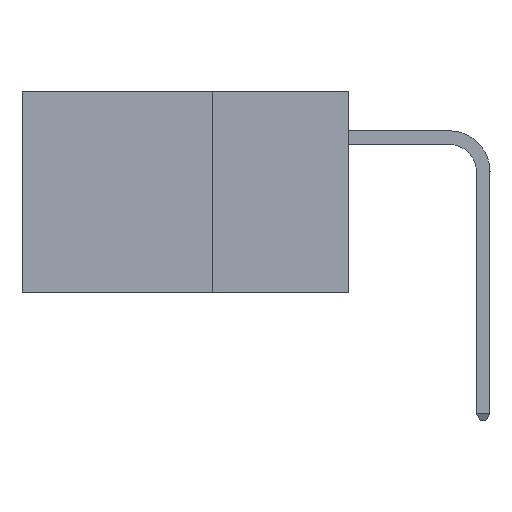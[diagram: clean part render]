
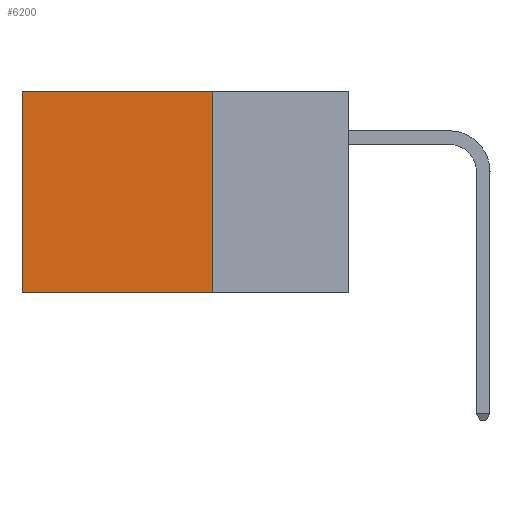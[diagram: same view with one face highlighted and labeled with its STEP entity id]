
A CAD part, left-side view. The second image highlights one B-rep face of the part: STEP entity #6200.
In plain terms, the highlighted planar face has unit normal (-1, 0, 0).
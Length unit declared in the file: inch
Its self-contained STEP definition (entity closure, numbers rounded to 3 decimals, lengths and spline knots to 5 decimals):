
#117 = VECTOR ( 'NONE', #3952, 39.37008 ) ;
#334 = PLANE ( 'NONE',  #3367 ) ;
#477 = FACE_OUTER_BOUND ( 'NONE', #5718, .T. ) ;
#944 = CARTESIAN_POINT ( 'NONE',  ( 0.2875, 0.25, 0. ) ) ;
#2582 = LINE ( 'NONE', #9122, #117 ) ;
#2603 = LINE ( 'NONE', #2713, #8702 ) ;
#2713 = CARTESIAN_POINT ( 'NONE',  ( 0.2875, 0.25, 0. ) ) ;
#2733 = CARTESIAN_POINT ( 'NONE',  ( 0.2875, 0.6, 0. ) ) ;
#2866 = LINE ( 'NONE', #10944, #5875 ) ;
#2928 = ORIENTED_EDGE ( 'NONE', *, *, #10273, .F. ) ;
#2999 = DIRECTION ( 'NONE',  ( 0., 0., -1. ) ) ;
#3357 = EDGE_CURVE ( 'NONE', #4830, #9668, #2582, .T. ) ;
#3367 = AXIS2_PLACEMENT_3D ( 'NONE', #944, #7029, #9924 ) ;
#3760 = ORIENTED_EDGE ( 'NONE', *, *, #9177, .T. ) ;
#3815 = CARTESIAN_POINT ( 'NONE',  ( 0.2875, 0.25, -0.37 ) ) ;
#3893 = ORIENTED_EDGE ( 'NONE', *, *, #7838, .F. ) ;
#3900 = DIRECTION ( 'NONE',  ( 0., 1., 0. ) ) ;
#3952 = DIRECTION ( 'NONE',  ( 0., 0., -1. ) ) ;
#4043 = ORIENTED_EDGE ( 'NONE', *, *, #3357, .T. ) ;
#4568 = DIRECTION ( 'NONE',  ( 0., 1., 0. ) ) ;
#4830 = VERTEX_POINT ( 'NONE', #2733 ) ;
#5718 = EDGE_LOOP ( 'NONE', ( #4043, #2928, #3893, #3760 ) ) ;
#5875 = VECTOR ( 'NONE', #3900, 39.37008 ) ;
#5929 = VECTOR ( 'NONE', #2999, 39.37008 ) ;
#6200 = ADVANCED_FACE ( 'NONE', ( #477 ), #334, .F. ) ;
#7029 = DIRECTION ( 'NONE',  ( 1., 0., 0. ) ) ;
#7339 = VERTEX_POINT ( 'NONE', #7905 ) ;
#7521 = VERTEX_POINT ( 'NONE', #3815 ) ;
#7642 = CARTESIAN_POINT ( 'NONE',  ( 0.2875, 0.6, -0.37 ) ) ;
#7838 = EDGE_CURVE ( 'NONE', #7339, #7521, #9569, .T. ) ;
#7905 = CARTESIAN_POINT ( 'NONE',  ( 0.2875, 0.25, 0. ) ) ;
#8702 = VECTOR ( 'NONE', #4568, 39.37008 ) ;
#9122 = CARTESIAN_POINT ( 'NONE',  ( 0.2875, 0.6, 0. ) ) ;
#9177 = EDGE_CURVE ( 'NONE', #7339, #4830, #2603, .T. ) ;
#9569 = LINE ( 'NONE', #10785, #5929 ) ;
#9668 = VERTEX_POINT ( 'NONE', #7642 ) ;
#9924 = DIRECTION ( 'NONE',  ( 0., 0., -1. ) ) ;
#10273 = EDGE_CURVE ( 'NONE', #7521, #9668, #2866, .T. ) ;
#10785 = CARTESIAN_POINT ( 'NONE',  ( 0.2875, 0.25, 0. ) ) ;
#10944 = CARTESIAN_POINT ( 'NONE',  ( 0.2875, 0.25, -0.37 ) ) ;
